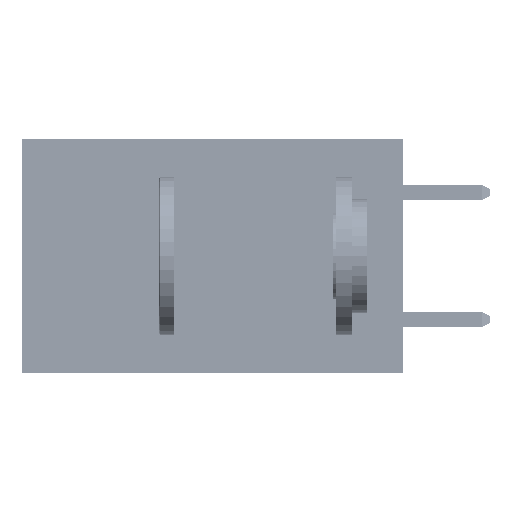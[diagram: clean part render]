
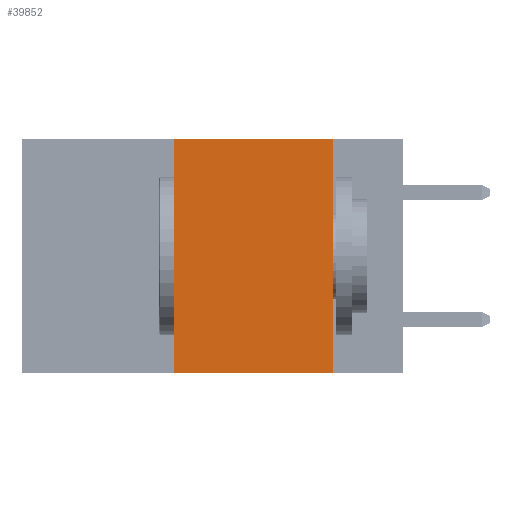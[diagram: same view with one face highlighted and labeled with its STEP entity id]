
A CAD part, left-side view. The second image highlights one B-rep face of the part: STEP entity #39852.
In plain terms, the highlighted planar face has unit normal (-1, 0, 0).
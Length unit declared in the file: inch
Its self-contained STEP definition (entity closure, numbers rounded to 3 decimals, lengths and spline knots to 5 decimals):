
#3775 = CARTESIAN_POINT ( 'NONE',  ( 0., 0.36, 0. ) ) ;
#3951 = CARTESIAN_POINT ( 'NONE',  ( 0., 0.36, -0.37 ) ) ;
#4933 = DIRECTION ( 'NONE',  ( 1., 0., 0. ) ) ;
#5097 = DIRECTION ( 'NONE',  ( 0., -1., 0. ) ) ;
#7166 = EDGE_LOOP ( 'NONE', ( #26136, #9356, #23088, #10920 ) ) ;
#9356 = ORIENTED_EDGE ( 'NONE', *, *, #30917, .F. ) ;
#9828 = AXIS2_PLACEMENT_3D ( 'NONE', #35054, #4933, #43082 ) ;
#10920 = ORIENTED_EDGE ( 'NONE', *, *, #46793, .T. ) ;
#14900 = EDGE_CURVE ( 'NONE', #17377, #48516, #34613, .T. ) ;
#15088 = LINE ( 'NONE', #38266, #16922 ) ;
#15475 = CARTESIAN_POINT ( 'NONE',  ( 0., 0.36, 0. ) ) ;
#15622 = DIRECTION ( 'NONE',  ( 0., -1., 0. ) ) ;
#16922 = VECTOR ( 'NONE', #15622, 39.37008 ) ;
#17377 = VERTEX_POINT ( 'NONE', #3951 ) ;
#18721 = CARTESIAN_POINT ( 'NONE',  ( 0., 0.11, 0. ) ) ;
#18763 = VECTOR ( 'NONE', #39054, 39.37008 ) ;
#19595 = LINE ( 'NONE', #42750, #48293 ) ;
#20077 = PLANE ( 'NONE',  #9828 ) ;
#23088 = ORIENTED_EDGE ( 'NONE', *, *, #14900, .F. ) ;
#23865 = VERTEX_POINT ( 'NONE', #18721 ) ;
#23928 = CARTESIAN_POINT ( 'NONE',  ( 0., 0.11, -0.37 ) ) ;
#24056 = CARTESIAN_POINT ( 'NONE',  ( 0., 0.11, 0. ) ) ;
#26136 = ORIENTED_EDGE ( 'NONE', *, *, #26268, .F. ) ;
#26268 = EDGE_CURVE ( 'NONE', #23865, #48630, #48663, .T. ) ;
#30917 = EDGE_CURVE ( 'NONE', #48516, #23865, #15088, .T. ) ;
#34613 = LINE ( 'NONE', #15475, #46572 ) ;
#35054 = CARTESIAN_POINT ( 'NONE',  ( 0., 0.6, 0. ) ) ;
#38266 = CARTESIAN_POINT ( 'NONE',  ( 0., 0.6, 0. ) ) ;
#38331 = DIRECTION ( 'NONE',  ( 0., 0., 1. ) ) ;
#39054 = DIRECTION ( 'NONE',  ( 0., 0., -1. ) ) ;
#39852 = ADVANCED_FACE ( 'NONE', ( #45766 ), #20077, .F. ) ;
#42750 = CARTESIAN_POINT ( 'NONE',  ( 0., 0.6, -0.37 ) ) ;
#43082 = DIRECTION ( 'NONE',  ( 0., 0., -1. ) ) ;
#45766 = FACE_OUTER_BOUND ( 'NONE', #7166, .T. ) ;
#46572 = VECTOR ( 'NONE', #38331, 39.37008 ) ;
#46793 = EDGE_CURVE ( 'NONE', #17377, #48630, #19595, .T. ) ;
#48293 = VECTOR ( 'NONE', #5097, 39.37008 ) ;
#48516 = VERTEX_POINT ( 'NONE', #3775 ) ;
#48630 = VERTEX_POINT ( 'NONE', #23928 ) ;
#48663 = LINE ( 'NONE', #24056, #18763 ) ;
